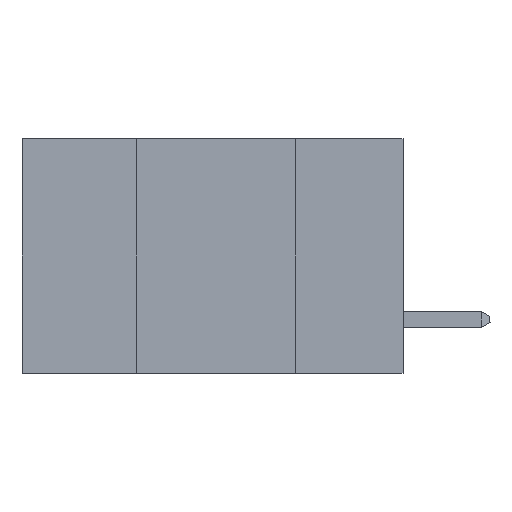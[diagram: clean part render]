
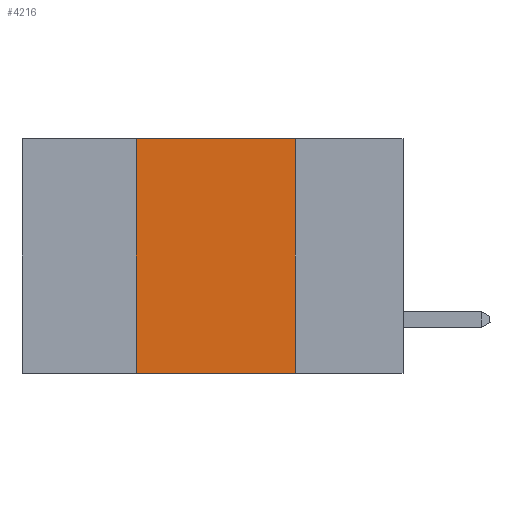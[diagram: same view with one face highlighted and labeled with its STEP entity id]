
A CAD part, left-side view. The second image highlights one B-rep face of the part: STEP entity #4216.
In plain terms, the highlighted planar face has unit normal (-1, 0, 0).
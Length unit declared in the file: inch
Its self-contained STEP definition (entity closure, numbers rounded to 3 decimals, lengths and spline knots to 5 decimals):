
#1 = VECTOR ( 'NONE', #27013, 39.37008 ) ;
#35 = EDGE_CURVE ( 'NONE', #4400, #17003, #37901, .T. ) ;
#596 = ORIENTED_EDGE ( 'NONE', *, *, #35, .F. ) ;
#2659 = CARTESIAN_POINT ( 'NONE',  ( 0., 0.17, 0. ) ) ;
#2798 = CARTESIAN_POINT ( 'NONE',  ( 0., 0.17, 0. ) ) ;
#4216 = ADVANCED_FACE ( 'NONE', ( #24378 ), #28617, .F. ) ;
#4400 = VERTEX_POINT ( 'NONE', #2798 ) ;
#4788 = CARTESIAN_POINT ( 'NONE',  ( 0., 0.42, 0. ) ) ;
#5512 = VERTEX_POINT ( 'NONE', #10971 ) ;
#6484 = CARTESIAN_POINT ( 'NONE',  ( 0., 0.6, -0.37 ) ) ;
#7331 = VECTOR ( 'NONE', #13291, 39.37008 ) ;
#8599 = ORIENTED_EDGE ( 'NONE', *, *, #20239, .F. ) ;
#9844 = CARTESIAN_POINT ( 'NONE',  ( 0., 0.17, -0.37 ) ) ;
#10971 = CARTESIAN_POINT ( 'NONE',  ( 0., 0.42, -0.37 ) ) ;
#11234 = CARTESIAN_POINT ( 'NONE',  ( 0., 0.42, 0. ) ) ;
#11498 = AXIS2_PLACEMENT_3D ( 'NONE', #32043, #38730, #25127 ) ;
#13291 = DIRECTION ( 'NONE',  ( 0., 0., 1. ) ) ;
#14509 = EDGE_CURVE ( 'NONE', #5512, #27815, #15331, .T. ) ;
#15331 = LINE ( 'NONE', #4788, #7331 ) ;
#17003 = VERTEX_POINT ( 'NONE', #9844 ) ;
#20239 = EDGE_CURVE ( 'NONE', #27815, #4400, #20658, .T. ) ;
#20658 = LINE ( 'NONE', #22750, #34052 ) ;
#22277 = EDGE_LOOP ( 'NONE', ( #596, #8599, #34266, #32920 ) ) ;
#22750 = CARTESIAN_POINT ( 'NONE',  ( 0., 0.6, 0. ) ) ;
#24378 = FACE_OUTER_BOUND ( 'NONE', #22277, .T. ) ;
#25127 = DIRECTION ( 'NONE',  ( 0., 0., -1. ) ) ;
#26180 = DIRECTION ( 'NONE',  ( 0., -1., 0. ) ) ;
#27013 = DIRECTION ( 'NONE',  ( 0., -1., 0. ) ) ;
#27815 = VERTEX_POINT ( 'NONE', #11234 ) ;
#28617 = PLANE ( 'NONE',  #11498 ) ;
#28895 = VECTOR ( 'NONE', #29776, 39.37008 ) ;
#29776 = DIRECTION ( 'NONE',  ( 0., 0., -1. ) ) ;
#32043 = CARTESIAN_POINT ( 'NONE',  ( 0., 0.6, 0. ) ) ;
#32920 = ORIENTED_EDGE ( 'NONE', *, *, #43502, .T. ) ;
#34052 = VECTOR ( 'NONE', #26180, 39.37008 ) ;
#34266 = ORIENTED_EDGE ( 'NONE', *, *, #14509, .F. ) ;
#37901 = LINE ( 'NONE', #2659, #28895 ) ;
#38730 = DIRECTION ( 'NONE',  ( 1., 0., 0. ) ) ;
#43151 = LINE ( 'NONE', #6484, #1 ) ;
#43502 = EDGE_CURVE ( 'NONE', #5512, #17003, #43151, .T. ) ;
